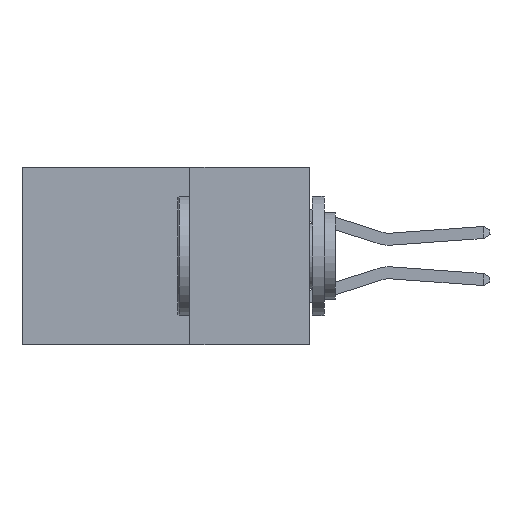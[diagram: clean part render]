
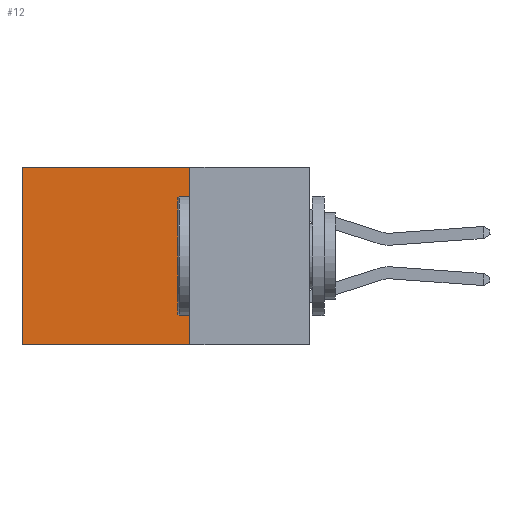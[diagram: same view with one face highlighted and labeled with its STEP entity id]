
A CAD part, left-side view. The second image highlights one B-rep face of the part: STEP entity #12.
In plain terms, the highlighted planar face has unit normal (-1, 0, 0).
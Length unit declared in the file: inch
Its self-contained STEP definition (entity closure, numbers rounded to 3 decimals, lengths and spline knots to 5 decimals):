
#12 = ADVANCED_FACE ( 'NONE', ( #916 ), #4349, .F. ) ;
#21 = LINE ( 'NONE', #3448, #12723 ) ;
#183 = CARTESIAN_POINT ( 'NONE',  ( 0.2615, 0.25, 0. ) ) ;
#258 = CARTESIAN_POINT ( 'NONE',  ( 0.2615, 0.6, -0.37 ) ) ;
#676 = CARTESIAN_POINT ( 'NONE',  ( 0.2615, 0.25, -0.37 ) ) ;
#916 = FACE_OUTER_BOUND ( 'NONE', #5056, .T. ) ;
#1337 = DIRECTION ( 'NONE',  ( 0., 0., -1. ) ) ;
#2224 = VECTOR ( 'NONE', #13291, 39.37008 ) ;
#2552 = AXIS2_PLACEMENT_3D ( 'NONE', #676, #13740, #10403 ) ;
#3142 = DIRECTION ( 'NONE',  ( 0., 1., 0. ) ) ;
#3448 = CARTESIAN_POINT ( 'NONE',  ( 0.2615, 0.25, 0. ) ) ;
#3605 = LINE ( 'NONE', #9654, #2224 ) ;
#4349 = PLANE ( 'NONE',  #2552 ) ;
#4483 = LINE ( 'NONE', #5421, #7831 ) ;
#5056 = EDGE_LOOP ( 'NONE', ( #15365, #5580, #13345, #14050 ) ) ;
#5421 = CARTESIAN_POINT ( 'NONE',  ( 0.2615, 0.25, -0.37 ) ) ;
#5580 = ORIENTED_EDGE ( 'NONE', *, *, #6277, .F. ) ;
#6277 = EDGE_CURVE ( 'NONE', #9883, #13209, #4483, .T. ) ;
#6866 = DIRECTION ( 'NONE',  ( 0., 1., 0. ) ) ;
#7831 = VECTOR ( 'NONE', #3142, 39.37008 ) ;
#7965 = CARTESIAN_POINT ( 'NONE',  ( 0.2615, 0.6, -0.37 ) ) ;
#8364 = CARTESIAN_POINT ( 'NONE',  ( 0.2615, 0.25, -0.37 ) ) ;
#9289 = EDGE_CURVE ( 'NONE', #15146, #13209, #12038, .T. ) ;
#9654 = CARTESIAN_POINT ( 'NONE',  ( 0.2615, 0.25, -0.37 ) ) ;
#9883 = VERTEX_POINT ( 'NONE', #8364 ) ;
#10260 = VECTOR ( 'NONE', #1337, 39.37008 ) ;
#10403 = DIRECTION ( 'NONE',  ( 0., 0., -1. ) ) ;
#10925 = VERTEX_POINT ( 'NONE', #183 ) ;
#11937 = EDGE_CURVE ( 'NONE', #10925, #9883, #3605, .T. ) ;
#12038 = LINE ( 'NONE', #258, #10260 ) ;
#12723 = VECTOR ( 'NONE', #6866, 39.37008 ) ;
#12856 = EDGE_CURVE ( 'NONE', #10925, #15146, #21, .T. ) ;
#13209 = VERTEX_POINT ( 'NONE', #7965 ) ;
#13291 = DIRECTION ( 'NONE',  ( 0., 0., -1. ) ) ;
#13345 = ORIENTED_EDGE ( 'NONE', *, *, #11937, .F. ) ;
#13740 = DIRECTION ( 'NONE',  ( 1., 0., 0. ) ) ;
#14050 = ORIENTED_EDGE ( 'NONE', *, *, #12856, .T. ) ;
#14990 = CARTESIAN_POINT ( 'NONE',  ( 0.2615, 0.6, 0. ) ) ;
#15146 = VERTEX_POINT ( 'NONE', #14990 ) ;
#15365 = ORIENTED_EDGE ( 'NONE', *, *, #9289, .T. ) ;
